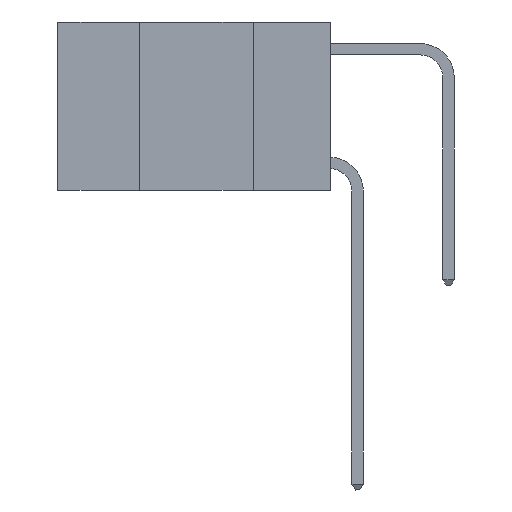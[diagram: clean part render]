
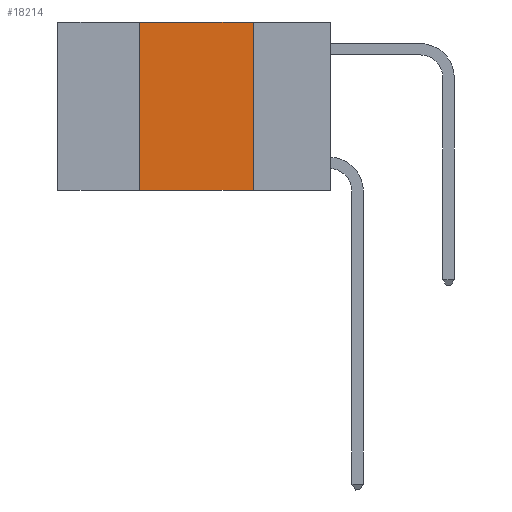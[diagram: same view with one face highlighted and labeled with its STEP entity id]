
A CAD part, left-side view. The second image highlights one B-rep face of the part: STEP entity #18214.
In plain terms, the highlighted planar face has unit normal (-1, 0, 0).
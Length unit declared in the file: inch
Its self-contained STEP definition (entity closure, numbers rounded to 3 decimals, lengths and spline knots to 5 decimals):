
#1291 = VECTOR ( 'NONE', #13130, 39.37008 ) ;
#1833 = DIRECTION ( 'NONE',  ( 0., 0., -1. ) ) ;
#2155 = DIRECTION ( 'NONE',  ( 1., 0., 0. ) ) ;
#2238 = VECTOR ( 'NONE', #1833, 39.37008 ) ;
#3228 = ORIENTED_EDGE ( 'NONE', *, *, #3340, .F. ) ;
#3340 = EDGE_CURVE ( 'NONE', #13534, #7177, #4697, .T. ) ;
#3579 = PLANE ( 'NONE',  #11770 ) ;
#4130 = EDGE_CURVE ( 'NONE', #5288, #18225, #15771, .T. ) ;
#4697 = LINE ( 'NONE', #10379, #2238 ) ;
#5288 = VERTEX_POINT ( 'NONE', #9065 ) ;
#6674 = VECTOR ( 'NONE', #9850, 39.37008 ) ;
#7083 = VECTOR ( 'NONE', #12823, 39.37008 ) ;
#7177 = VERTEX_POINT ( 'NONE', #12083 ) ;
#7210 = CARTESIAN_POINT ( 'NONE',  ( 0., 0.42, 0. ) ) ;
#7774 = FACE_OUTER_BOUND ( 'NONE', #15890, .T. ) ;
#8580 = LINE ( 'NONE', #14258, #7083 ) ;
#9065 = CARTESIAN_POINT ( 'NONE',  ( 0., 0.42, -0.37 ) ) ;
#9234 = CARTESIAN_POINT ( 'NONE',  ( 0., 0.17, 0. ) ) ;
#9263 = DIRECTION ( 'NONE',  ( 0., 0., -1. ) ) ;
#9850 = DIRECTION ( 'NONE',  ( 0., -1., 0. ) ) ;
#9853 = CARTESIAN_POINT ( 'NONE',  ( 0., 0.42, 0. ) ) ;
#9949 = ORIENTED_EDGE ( 'NONE', *, *, #4130, .F. ) ;
#10379 = CARTESIAN_POINT ( 'NONE',  ( 0., 0.17, 0. ) ) ;
#11516 = ORIENTED_EDGE ( 'NONE', *, *, #14623, .F. ) ;
#11770 = AXIS2_PLACEMENT_3D ( 'NONE', #16162, #2155, #9263 ) ;
#11901 = ORIENTED_EDGE ( 'NONE', *, *, #17357, .T. ) ;
#12083 = CARTESIAN_POINT ( 'NONE',  ( 0., 0.17, -0.37 ) ) ;
#12823 = DIRECTION ( 'NONE',  ( 0., -1., 0. ) ) ;
#13130 = DIRECTION ( 'NONE',  ( 0., 0., 1. ) ) ;
#13534 = VERTEX_POINT ( 'NONE', #9234 ) ;
#14258 = CARTESIAN_POINT ( 'NONE',  ( 0., 0.6, -0.37 ) ) ;
#14623 = EDGE_CURVE ( 'NONE', #18225, #13534, #15612, .T. ) ;
#15612 = LINE ( 'NONE', #18294, #6674 ) ;
#15771 = LINE ( 'NONE', #7210, #1291 ) ;
#15890 = EDGE_LOOP ( 'NONE', ( #3228, #11516, #9949, #11901 ) ) ;
#16162 = CARTESIAN_POINT ( 'NONE',  ( 0., 0.6, 0. ) ) ;
#17357 = EDGE_CURVE ( 'NONE', #5288, #7177, #8580, .T. ) ;
#18214 = ADVANCED_FACE ( 'NONE', ( #7774 ), #3579, .F. ) ;
#18225 = VERTEX_POINT ( 'NONE', #9853 ) ;
#18294 = CARTESIAN_POINT ( 'NONE',  ( 0., 0.6, 0. ) ) ;
